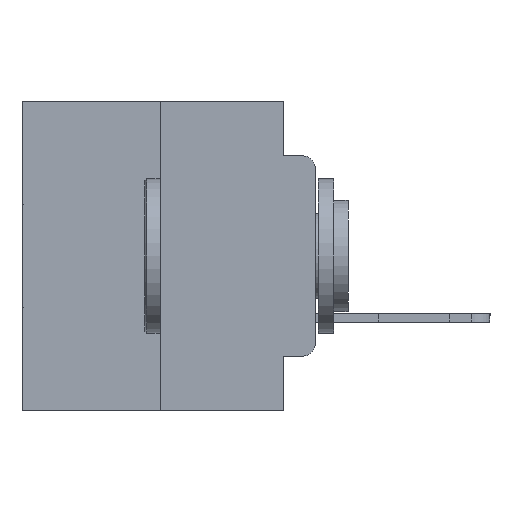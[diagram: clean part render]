
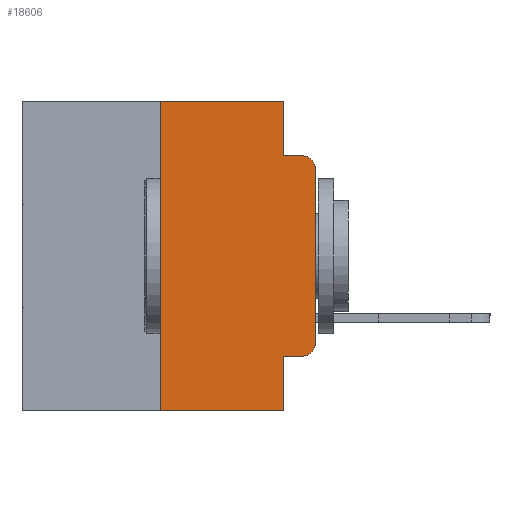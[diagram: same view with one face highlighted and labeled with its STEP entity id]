
A CAD part, left-side view. The second image highlights one B-rep face of the part: STEP entity #18606.
In plain terms, the highlighted planar face has unit normal (-1, 0, 0).
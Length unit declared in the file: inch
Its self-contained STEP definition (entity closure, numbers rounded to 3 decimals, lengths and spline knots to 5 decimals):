
#274 = LINE ( 'NONE', #10407, #10781 ) ;
#307 = ORIENTED_EDGE ( 'NONE', *, *, #24425, .F. ) ;
#393 = CARTESIAN_POINT ( 'NONE',  ( 0., 0., -0.1085 ) ) ;
#841 = CARTESIAN_POINT ( 'NONE',  ( 0., 0.051, -0.4115 ) ) ;
#937 = ORIENTED_EDGE ( 'NONE', *, *, #2699, .F. ) ;
#1213 = DIRECTION ( 'NONE',  ( 0., -1., 0. ) ) ;
#1548 = VECTOR ( 'NONE', #15331, 39.37008 ) ;
#1638 = DIRECTION ( 'NONE',  ( 0., -1., 0. ) ) ;
#1955 = DIRECTION ( 'NONE',  ( 0., 0., -1. ) ) ;
#2234 = CIRCLE ( 'NONE', #5728, 0.02 ) ;
#2291 = ORIENTED_EDGE ( 'NONE', *, *, #8280, .T. ) ;
#2418 = VERTEX_POINT ( 'NONE', #26796 ) ;
#2484 = CARTESIAN_POINT ( 'NONE',  ( 0., 0.02, -0.3915 ) ) ;
#2699 = EDGE_CURVE ( 'NONE', #10110, #8311, #24071, .T. ) ;
#3250 = ORIENTED_EDGE ( 'NONE', *, *, #15716, .F. ) ;
#3332 = ORIENTED_EDGE ( 'NONE', *, *, #18773, .T. ) ;
#3795 = CARTESIAN_POINT ( 'NONE',  ( 0., 0.051, -0.0885 ) ) ;
#4114 = EDGE_CURVE ( 'NONE', #6123, #8311, #2234, .T. ) ;
#4379 = DIRECTION ( 'NONE',  ( 0., 0., 1. ) ) ;
#4455 = LINE ( 'NONE', #19301, #20614 ) ;
#4594 = DIRECTION ( 'NONE',  ( 0., 0., -1. ) ) ;
#5070 = LINE ( 'NONE', #15958, #15624 ) ;
#5220 = CARTESIAN_POINT ( 'NONE',  ( 0., 0.051, 0. ) ) ;
#5418 = VERTEX_POINT ( 'NONE', #12724 ) ;
#5512 = EDGE_CURVE ( 'NONE', #5418, #6123, #4455, .T. ) ;
#5728 = AXIS2_PLACEMENT_3D ( 'NONE', #27184, #14582, #1955 ) ;
#6123 = VERTEX_POINT ( 'NONE', #393 ) ;
#6389 = VECTOR ( 'NONE', #9273, 39.37008 ) ;
#7193 = EDGE_LOOP ( 'NONE', ( #17421, #24338, #937, #11820, #3250, #307, #2291, #8255, #24773, #3332 ) ) ;
#7562 = CARTESIAN_POINT ( 'NONE',  ( 0., 0.02, -0.0885 ) ) ;
#8161 = VERTEX_POINT ( 'NONE', #841 ) ;
#8201 = CARTESIAN_POINT ( 'NONE',  ( 0., 0.473, 0. ) ) ;
#8255 = ORIENTED_EDGE ( 'NONE', *, *, #23026, .F. ) ;
#8280 = EDGE_CURVE ( 'NONE', #9817, #26463, #5070, .T. ) ;
#8311 = VERTEX_POINT ( 'NONE', #7562 ) ;
#9257 = VERTEX_POINT ( 'NONE', #5220 ) ;
#9273 = DIRECTION ( 'NONE',  ( 0., 0., -1. ) ) ;
#9332 = CARTESIAN_POINT ( 'NONE',  ( 0., 0.051, -0.5 ) ) ;
#9817 = VERTEX_POINT ( 'NONE', #17565 ) ;
#10110 = VERTEX_POINT ( 'NONE', #14335 ) ;
#10407 = CARTESIAN_POINT ( 'NONE',  ( 0., 0.051, 0. ) ) ;
#10781 = VECTOR ( 'NONE', #23068, 39.37008 ) ;
#11096 = DIRECTION ( 'NONE',  ( 0., -1., 0. ) ) ;
#11807 = DIRECTION ( 'NONE',  ( 0., -1., 0. ) ) ;
#11820 = ORIENTED_EDGE ( 'NONE', *, *, #25821, .F. ) ;
#12434 = DIRECTION ( 'NONE',  ( 0., 0., -1. ) ) ;
#12498 = VECTOR ( 'NONE', #11807, 39.37008 ) ;
#12724 = CARTESIAN_POINT ( 'NONE',  ( 0., 0., -0.3915 ) ) ;
#12870 = AXIS2_PLACEMENT_3D ( 'NONE', #8201, #25063, #12434 ) ;
#14251 = CARTESIAN_POINT ( 'NONE',  ( 0., 0.473, 0. ) ) ;
#14280 = CARTESIAN_POINT ( 'NONE',  ( 0., 0.02, -0.4115 ) ) ;
#14335 = CARTESIAN_POINT ( 'NONE',  ( 0., 0.051, -0.0885 ) ) ;
#14582 = DIRECTION ( 'NONE',  ( -1., 0., 0. ) ) ;
#15241 = CIRCLE ( 'NONE', #24193, 0.02 ) ;
#15331 = DIRECTION ( 'NONE',  ( 0., 0., 1. ) ) ;
#15624 = VECTOR ( 'NONE', #1213, 39.37008 ) ;
#15658 = CARTESIAN_POINT ( 'NONE',  ( 0., 0.051, 0. ) ) ;
#15716 = EDGE_CURVE ( 'NONE', #2418, #9257, #21309, .T. ) ;
#15958 = CARTESIAN_POINT ( 'NONE',  ( 0., 0.473, -0.5 ) ) ;
#16959 = LINE ( 'NONE', #15658, #6389 ) ;
#17025 = VECTOR ( 'NONE', #1638, 39.37008 ) ;
#17229 = DIRECTION ( 'NONE',  ( -1., 0., 0. ) ) ;
#17421 = ORIENTED_EDGE ( 'NONE', *, *, #5512, .T. ) ;
#17565 = CARTESIAN_POINT ( 'NONE',  ( 0., 0.25, -0.5 ) ) ;
#18359 = LINE ( 'NONE', #25814, #1548 ) ;
#18606 = ADVANCED_FACE ( 'NONE', ( #19212 ), #27090, .F. ) ;
#18773 = EDGE_CURVE ( 'NONE', #23494, #5418, #15241, .T. ) ;
#19212 = FACE_OUTER_BOUND ( 'NONE', #7193, .T. ) ;
#19301 = CARTESIAN_POINT ( 'NONE',  ( 0., 0., 0. ) ) ;
#20168 = EDGE_CURVE ( 'NONE', #8161, #23494, #23086, .T. ) ;
#20614 = VECTOR ( 'NONE', #4379, 39.37008 ) ;
#21309 = LINE ( 'NONE', #14251, #17025 ) ;
#22352 = CARTESIAN_POINT ( 'NONE',  ( 0., 0.051, -0.4115 ) ) ;
#23026 = EDGE_CURVE ( 'NONE', #8161, #26463, #274, .T. ) ;
#23068 = DIRECTION ( 'NONE',  ( 0., 0., -1. ) ) ;
#23086 = LINE ( 'NONE', #22352, #12498 ) ;
#23417 = VECTOR ( 'NONE', #11096, 39.37008 ) ;
#23494 = VERTEX_POINT ( 'NONE', #14280 ) ;
#24071 = LINE ( 'NONE', #3795, #23417 ) ;
#24193 = AXIS2_PLACEMENT_3D ( 'NONE', #2484, #17229, #4594 ) ;
#24338 = ORIENTED_EDGE ( 'NONE', *, *, #4114, .T. ) ;
#24425 = EDGE_CURVE ( 'NONE', #9817, #2418, #18359, .T. ) ;
#24773 = ORIENTED_EDGE ( 'NONE', *, *, #20168, .T. ) ;
#25063 = DIRECTION ( 'NONE',  ( 1., 0., 0. ) ) ;
#25814 = CARTESIAN_POINT ( 'NONE',  ( 0., 0.25, 0. ) ) ;
#25821 = EDGE_CURVE ( 'NONE', #9257, #10110, #16959, .T. ) ;
#26463 = VERTEX_POINT ( 'NONE', #9332 ) ;
#26796 = CARTESIAN_POINT ( 'NONE',  ( 0., 0.25, 0. ) ) ;
#27090 = PLANE ( 'NONE',  #12870 ) ;
#27184 = CARTESIAN_POINT ( 'NONE',  ( 0., 0.02, -0.1085 ) ) ;
